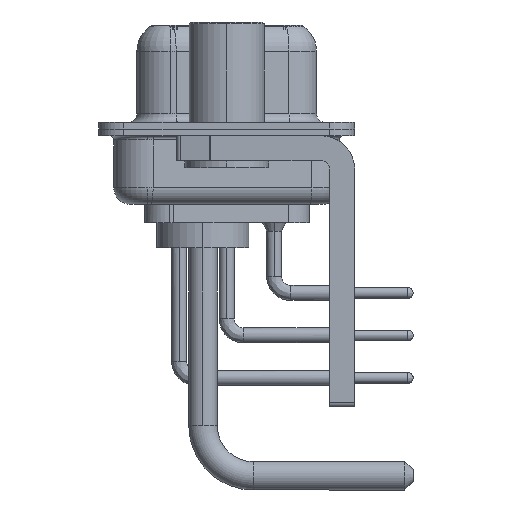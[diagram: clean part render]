
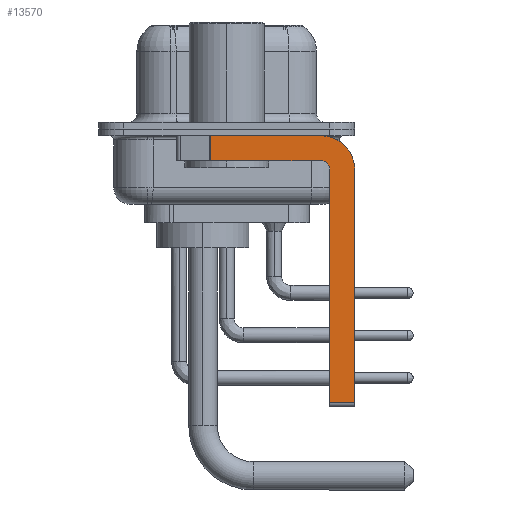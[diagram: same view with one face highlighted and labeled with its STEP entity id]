
A CAD part, left-side view. The second image highlights one B-rep face of the part: STEP entity #13570.
In plain terms, the highlighted planar face has unit normal (-1, 0, 0).
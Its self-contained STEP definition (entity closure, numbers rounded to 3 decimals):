
#1229 = EDGE_CURVE ( 'NONE', #35009, #17112, #24180, .T. ) ;
#1328 = EDGE_CURVE ( 'NONE', #15142, #20454, #27659, .T. ) ;
#1397 = VECTOR ( 'NONE', #17250, 1000. ) ;
#1827 = AXIS2_PLACEMENT_3D ( 'NONE', #8080, #13418, #27196 ) ;
#2689 = DIRECTION ( 'NONE',  ( -1., 0., 0. ) ) ;
#3329 = EDGE_LOOP ( 'NONE', ( #14423, #16919, #26395, #9627, #5152, #4770, #34214, #23504 ) ) ;
#4453 = DIRECTION ( 'NONE',  ( 0., -1., 0. ) ) ;
#4770 = ORIENTED_EDGE ( 'NONE', *, *, #1328, .T. ) ;
#5152 = ORIENTED_EDGE ( 'NONE', *, *, #21575, .F. ) ;
#5362 = AXIS2_PLACEMENT_3D ( 'NONE', #16033, #16715, #11071 ) ;
#6630 = LINE ( 'NONE', #14965, #1397 ) ;
#6867 = DIRECTION ( 'NONE',  ( 0., 0., 1. ) ) ;
#6926 = CIRCLE ( 'NONE', #1827, 2. ) ;
#7388 = VERTEX_POINT ( 'NONE', #26569 ) ;
#8080 = CARTESIAN_POINT ( 'NONE',  ( -2.9, -5.65, -2.4 ) ) ;
#9627 = ORIENTED_EDGE ( 'NONE', *, *, #1229, .F. ) ;
#11071 = DIRECTION ( 'NONE',  ( 0., 0., -1. ) ) ;
#11254 = PLANE ( 'NONE',  #5362 ) ;
#13418 = DIRECTION ( 'NONE',  ( 1., 0., 0. ) ) ;
#13535 = DIRECTION ( 'NONE',  ( 0., 0., 1. ) ) ;
#13570 = ADVANCED_FACE ( 'NONE', ( #19217 ), #11254, .F. ) ;
#13691 = VECTOR ( 'NONE', #6867, 1000. ) ;
#14036 = AXIS2_PLACEMENT_3D ( 'NONE', #31586, #2689, #13535 ) ;
#14423 = ORIENTED_EDGE ( 'NONE', *, *, #15760, .F. ) ;
#14573 = EDGE_CURVE ( 'NONE', #17112, #16249, #27617, .T. ) ;
#14965 = CARTESIAN_POINT ( 'NONE',  ( -2.9, -7.65, -2.4 ) ) ;
#15048 = EDGE_CURVE ( 'NONE', #7388, #20454, #6630, .T. ) ;
#15101 = CARTESIAN_POINT ( 'NONE',  ( -2.9, 3., -0.4 ) ) ;
#15142 = VERTEX_POINT ( 'NONE', #30357 ) ;
#15760 = EDGE_CURVE ( 'NONE', #20581, #18369, #25862, .T. ) ;
#16033 = CARTESIAN_POINT ( 'NONE',  ( -2.9, -5.65, -2.4 ) ) ;
#16249 = VERTEX_POINT ( 'NONE', #26873 ) ;
#16508 = CARTESIAN_POINT ( 'NONE',  ( -2.9, -5.65, -16.35 ) ) ;
#16715 = DIRECTION ( 'NONE',  ( 1., 0., 0. ) ) ;
#16919 = ORIENTED_EDGE ( 'NONE', *, *, #21772, .T. ) ;
#17110 = VECTOR ( 'NONE', #31994, 1000. ) ;
#17112 = VERTEX_POINT ( 'NONE', #26216 ) ;
#17250 = DIRECTION ( 'NONE',  ( 0., 0., -1. ) ) ;
#18274 = CARTESIAN_POINT ( 'NONE',  ( -2.9, 0.978, -0.4 ) ) ;
#18369 = VERTEX_POINT ( 'NONE', #27214 ) ;
#19217 = FACE_OUTER_BOUND ( 'NONE', #3329, .T. ) ;
#20107 = VECTOR ( 'NONE', #4453, 1000. ) ;
#20336 = CARTESIAN_POINT ( 'NONE',  ( -2.9, -6.15, -16.6 ) ) ;
#20454 = VERTEX_POINT ( 'NONE', #20576 ) ;
#20576 = CARTESIAN_POINT ( 'NONE',  ( -2.9, -7.65, -16.35 ) ) ;
#20581 = VERTEX_POINT ( 'NONE', #18274 ) ;
#21575 = EDGE_CURVE ( 'NONE', #15142, #35009, #25270, .T. ) ;
#21728 = VECTOR ( 'NONE', #28141, 1000. ) ;
#21772 = EDGE_CURVE ( 'NONE', #20581, #16249, #29338, .T. ) ;
#21879 = EDGE_CURVE ( 'NONE', #18369, #7388, #6926, .T. ) ;
#23504 = ORIENTED_EDGE ( 'NONE', *, *, #21879, .F. ) ;
#24180 = CIRCLE ( 'NONE', #14036, 0.5 ) ;
#25270 = LINE ( 'NONE', #20336, #13691 ) ;
#25862 = LINE ( 'NONE', #15101, #20107 ) ;
#26216 = CARTESIAN_POINT ( 'NONE',  ( -2.9, -5.65, -1.9 ) ) ;
#26395 = ORIENTED_EDGE ( 'NONE', *, *, #14573, .F. ) ;
#26569 = CARTESIAN_POINT ( 'NONE',  ( -2.9, -7.65, -2.4 ) ) ;
#26873 = CARTESIAN_POINT ( 'NONE',  ( -2.9, 0.978, -1.9 ) ) ;
#27196 = DIRECTION ( 'NONE',  ( 0., 0., -1. ) ) ;
#27214 = CARTESIAN_POINT ( 'NONE',  ( -2.9, -5.65, -0.4 ) ) ;
#27617 = LINE ( 'NONE', #30082, #21728 ) ;
#27659 = LINE ( 'NONE', #16508, #33825 ) ;
#28141 = DIRECTION ( 'NONE',  ( 0., 1., 0. ) ) ;
#29338 = LINE ( 'NONE', #31652, #17110 ) ;
#30082 = CARTESIAN_POINT ( 'NONE',  ( -2.9, -5.65, -1.9 ) ) ;
#30357 = CARTESIAN_POINT ( 'NONE',  ( -2.9, -6.15, -16.35 ) ) ;
#31586 = CARTESIAN_POINT ( 'NONE',  ( -2.9, -5.65, -2.4 ) ) ;
#31652 = CARTESIAN_POINT ( 'NONE',  ( -2.9, 0.978, -1.9 ) ) ;
#31994 = DIRECTION ( 'NONE',  ( 0., 0., -1. ) ) ;
#32968 = DIRECTION ( 'NONE',  ( 0., -1., 0. ) ) ;
#33825 = VECTOR ( 'NONE', #32968, 1000. ) ;
#34214 = ORIENTED_EDGE ( 'NONE', *, *, #15048, .F. ) ;
#34329 = CARTESIAN_POINT ( 'NONE',  ( -2.9, -6.15, -2.4 ) ) ;
#35009 = VERTEX_POINT ( 'NONE', #34329 ) ;
